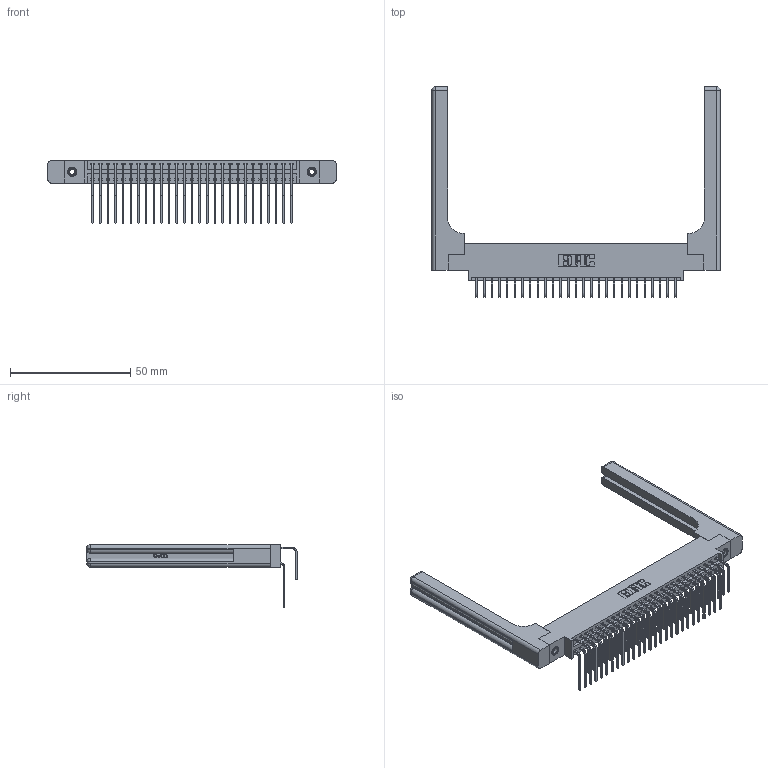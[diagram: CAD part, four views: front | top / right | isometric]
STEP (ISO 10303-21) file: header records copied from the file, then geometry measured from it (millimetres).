
FILE_DESCRIPTION (( 'STEP AP203' ), '1' );
FILE_NAME ('396-054-558-858.STEP', '2019-11-03T09:04:01', ( '' ), ( '' ), 'SwSTEP 2.0', 'SolidWorks 2016', '' );
FILE_SCHEMA (( 'CONFIG_CONTROL_DESIGN' ));
Length unit declared in the file: inch
Products named in the file (6): 345-250-001_345-250-001-102; 346 Part_0.170 Offset - 0.156 Dia-TH; 345-292-001_558 559 Tail - 1; 345-292-001_558 Tail - 2; 346-220-058_345-220-058; 396-054-558-858
Assembly tree (59 placements, depth 2):
  396-054-558-858
    346 Part_0.170 Offset - 0.156 Dia-TH
    345-292-001_558 559 Tail - 1  x27
    345-292-001_558 Tail - 2  x27
    345-250-001_345-250-001-102  x2
    346-220-058_345-220-058  x2
Bounding box: 119.79 x 87.44 x 26.16 mm (x, y, z)
Volume: 19215.3 mm3; surface area: 22522.5 mm2
Topology: 59 solids, 59 shells, 3298 faces, 9701 edges, 6374 vertices
Faces by surface type: plane 2226, cylinder 1012, bspline 36, cone 12, sphere 8, torus 4
Entity records: 26738 total; most frequent: CARTESIAN_POINT 5488, ORIENTED_EDGE 4168, DIRECTION 3792, EDGE_CURVE 2084, LINE 1712, VECTOR 1712, VERTEX_POINT 1378, AXIS2_PLACEMENT_3D 1040
